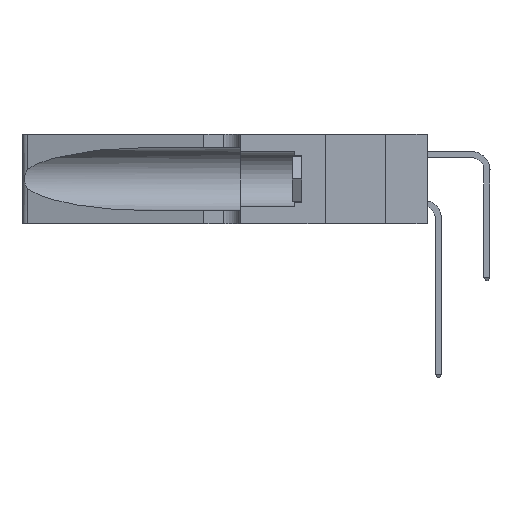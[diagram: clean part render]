
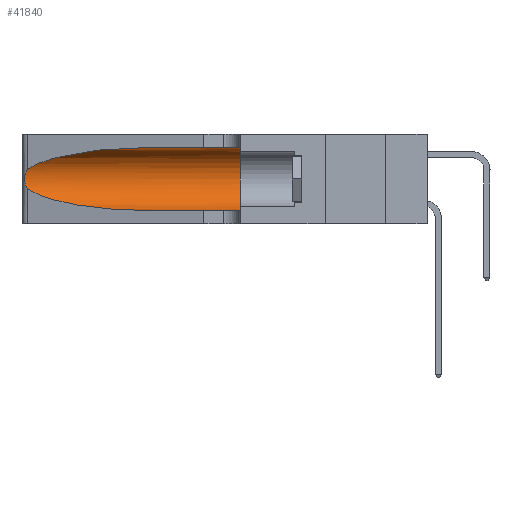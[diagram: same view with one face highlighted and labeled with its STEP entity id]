
A CAD part, left-side view. The second image highlights one B-rep face of the part: STEP entity #41840.
In plain terms, the highlighted cylindrical face has radius 3.308 mm (diameter 6.617 mm), a partial arc.
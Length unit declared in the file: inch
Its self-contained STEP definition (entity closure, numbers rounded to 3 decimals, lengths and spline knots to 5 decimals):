
#78 = CARTESIAN_POINT ( 'NONE',  ( 0.1305, 1.61858, 0.185 ) ) ;
#914 = CARTESIAN_POINT ( 'NONE',  ( 0.26017, 1.23833, 0.17102 ) ) ;
#1381 = EDGE_CURVE ( 'NONE', #16558, #34636, #10670, .T. ) ;
#1959 = B_SPLINE_CURVE_WITH_KNOTS ( 'NONE', 3,
 ( #22505, #18838, #36886, #15425, #40506, #19001, #44097, #22653, #914, #26262, #4610, #29880, #8281, #33445 ),
 .UNSPECIFIED., .F., .F.,
 ( 4, 2, 2, 2, 2, 2, 4 ),
 ( 0., 0.00027, 0.00053, 0.00107, 0.0016, 0.00187, 0.00214 ),
 .UNSPECIFIED. ) ;
#2604 = EDGE_CURVE ( 'NONE', #41111, #21414, #13951, .T. ) ;
#3159 = DIRECTION ( 'NONE',  ( 0., -1., 0. ) ) ;
#4610 = CARTESIAN_POINT ( 'NONE',  ( 0.25789, 1.23486, 0.15765 ) ) ;
#5205 = CARTESIAN_POINT ( 'NONE',  ( 0.1305, 0.35, 0.185 ) ) ;
#7448 = DIRECTION ( 'NONE',  ( 0., -1., 0. ) ) ;
#7704 = DIRECTION ( 'NONE',  ( 0., -1., 0. ) ) ;
#8281 = CARTESIAN_POINT ( 'NONE',  ( 0.25555, 1.22993, 0.14849 ) ) ;
#8883 = DIRECTION ( 'NONE',  ( 0., 0., 1. ) ) ;
#9488 = CARTESIAN_POINT ( 'NONE',  ( 0.18966, 0.96281, 0.31525 ) ) ;
#9542 = VECTOR ( 'NONE', #7704, 39.37008 ) ;
#10327 = EDGE_CURVE ( 'NONE', #34636, #15665, #16838, .T. ) ;
#10670 = LINE ( 'NONE', #40104, #9542 ) ;
#11872 = ORIENTED_EDGE ( 'NONE', *, *, #14237, .T. ) ;
#11897 =( BOUNDED_CURVE ( )  B_SPLINE_CURVE ( 3, ( #38268, #9488, #41873, #20400 ),
 .UNSPECIFIED., .F., .F. ) 
 B_SPLINE_CURVE_WITH_KNOTS ( ( 4, 4 ),
 ( 1.5708, 2.84003 ),
 .UNSPECIFIED. ) 
 CURVE ( )  GEOMETRIC_REPRESENTATION_ITEM ( )  RATIONAL_B_SPLINE_CURVE ( ( 1., 0.87, 0.87, 1. ) ) 
 REPRESENTATION_ITEM ( '' )  );
#12579 = ORIENTED_EDGE ( 'NONE', *, *, #10327, .F. ) ;
#13951 =( BOUNDED_CURVE ( )  B_SPLINE_CURVE ( 3, ( #35933, #39550, #14467, #43146 ),
 .UNSPECIFIED., .F., .T. ) 
 B_SPLINE_CURVE_WITH_KNOTS ( ( 4, 4 ),
 ( 3.44316, 4.71239 ),
 .UNSPECIFIED. ) 
 CURVE ( )  GEOMETRIC_REPRESENTATION_ITEM ( )  RATIONAL_B_SPLINE_CURVE ( ( 1., 0.87, 0.87, 1. ) ) 
 REPRESENTATION_ITEM ( '' )  );
#14169 = LINE ( 'NONE', #46278, #32140 ) ;
#14237 = EDGE_CURVE ( 'NONE', #29055, #41111, #1959, .T. ) ;
#14467 = CARTESIAN_POINT ( 'NONE',  ( 0.18966, 0.96281, 0.05475 ) ) ;
#15425 = CARTESIAN_POINT ( 'NONE',  ( 0.25787, 1.23484, 0.2124 ) ) ;
#15665 = VERTEX_POINT ( 'NONE', #23788 ) ;
#16177 = CYLINDRICAL_SURFACE ( 'NONE', #45418, 0.13025 ) ;
#16558 = VERTEX_POINT ( 'NONE', #30733 ) ;
#16838 = CIRCLE ( 'NONE', #25219, 0.13025 ) ;
#17514 = EDGE_CURVE ( 'NONE', #21414, #15665, #14169, .T. ) ;
#18199 = DIRECTION ( 'NONE',  ( 0., 0., -1. ) ) ;
#18838 = CARTESIAN_POINT ( 'NONE',  ( 0.25555, 1.22994, 0.2215 ) ) ;
#18857 = EDGE_LOOP ( 'NONE', ( #29152, #11872, #27351, #28313, #12579, #30418 ) ) ;
#19001 = CARTESIAN_POINT ( 'NONE',  ( 0.26018, 1.23835, 0.19895 ) ) ;
#20400 = CARTESIAN_POINT ( 'NONE',  ( 0.25487, 1.22718, 0.22369 ) ) ;
#21414 = VERTEX_POINT ( 'NONE', #35385 ) ;
#22505 = CARTESIAN_POINT ( 'NONE',  ( 0.25487, 1.22718, 0.22369 ) ) ;
#22653 = CARTESIAN_POINT ( 'NONE',  ( 0.26075, 1.23896, 0.178 ) ) ;
#23777 = CARTESIAN_POINT ( 'NONE',  ( 0.25487, 1.22718, 0.22369 ) ) ;
#23788 = CARTESIAN_POINT ( 'NONE',  ( 0.1305, 0.35, 0.05475 ) ) ;
#25219 = AXIS2_PLACEMENT_3D ( 'NONE', #5205, #30477, #8883 ) ;
#26262 = CARTESIAN_POINT ( 'NONE',  ( 0.25856, 1.23593, 0.16098 ) ) ;
#27351 = ORIENTED_EDGE ( 'NONE', *, *, #2604, .T. ) ;
#28313 = ORIENTED_EDGE ( 'NONE', *, *, #17514, .T. ) ;
#29055 = VERTEX_POINT ( 'NONE', #23777 ) ;
#29152 = ORIENTED_EDGE ( 'NONE', *, *, #43645, .T. ) ;
#29880 = CARTESIAN_POINT ( 'NONE',  ( 0.25639, 1.23186, 0.15144 ) ) ;
#30418 = ORIENTED_EDGE ( 'NONE', *, *, #1381, .F. ) ;
#30477 = DIRECTION ( 'NONE',  ( 0., 1., 0. ) ) ;
#30733 = CARTESIAN_POINT ( 'NONE',  ( 0.1305, 0.72297, 0.31525 ) ) ;
#32140 = VECTOR ( 'NONE', #3159, 39.37008 ) ;
#33445 = CARTESIAN_POINT ( 'NONE',  ( 0.25487, 1.22718, 0.14631 ) ) ;
#34636 = VERTEX_POINT ( 'NONE', #45501 ) ;
#35385 = CARTESIAN_POINT ( 'NONE',  ( 0.1305, 0.72297, 0.05475 ) ) ;
#35933 = CARTESIAN_POINT ( 'NONE',  ( 0.25487, 1.22718, 0.14631 ) ) ;
#36367 = FACE_OUTER_BOUND ( 'NONE', #18857, .T. ) ;
#36886 = CARTESIAN_POINT ( 'NONE',  ( 0.25639, 1.23184, 0.21858 ) ) ;
#38268 = CARTESIAN_POINT ( 'NONE',  ( 0.1305, 0.72297, 0.31525 ) ) ;
#39550 = CARTESIAN_POINT ( 'NONE',  ( 0.2373, 1.15595, 0.08982 ) ) ;
#39609 = CARTESIAN_POINT ( 'NONE',  ( 0.25487, 1.22718, 0.14631 ) ) ;
#40104 = CARTESIAN_POINT ( 'NONE',  ( 0.1305, 1.61858, 0.31525 ) ) ;
#40506 = CARTESIAN_POINT ( 'NONE',  ( 0.25854, 1.2359, 0.20912 ) ) ;
#41111 = VERTEX_POINT ( 'NONE', #39609 ) ;
#41840 = ADVANCED_FACE ( 'NONE', ( #36367 ), #16177, .F. ) ;
#41873 = CARTESIAN_POINT ( 'NONE',  ( 0.2373, 1.15595, 0.28018 ) ) ;
#43146 = CARTESIAN_POINT ( 'NONE',  ( 0.1305, 0.72297, 0.05475 ) ) ;
#43645 = EDGE_CURVE ( 'NONE', #16558, #29055, #11897, .T. ) ;
#44097 = CARTESIAN_POINT ( 'NONE',  ( 0.26075, 1.23896, 0.19203 ) ) ;
#45418 = AXIS2_PLACEMENT_3D ( 'NONE', #78, #7448, #18199 ) ;
#45501 = CARTESIAN_POINT ( 'NONE',  ( 0.1305, 0.35, 0.31525 ) ) ;
#46278 = CARTESIAN_POINT ( 'NONE',  ( 0.1305, 1.61858, 0.05475 ) ) ;
